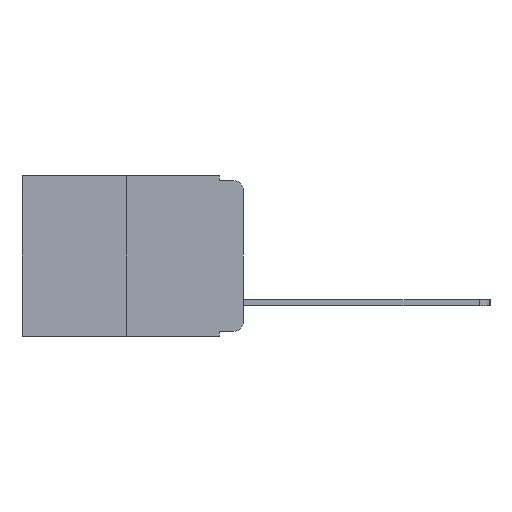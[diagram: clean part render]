
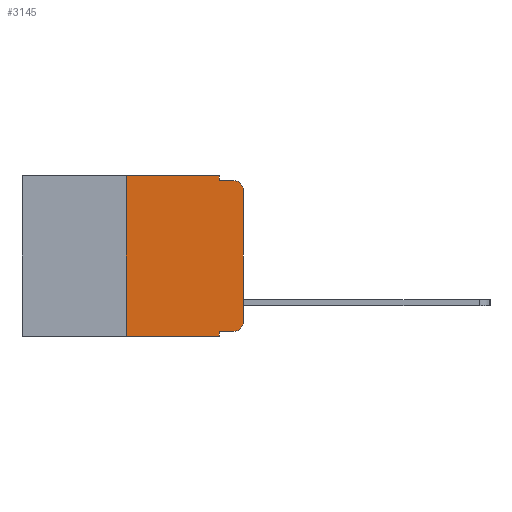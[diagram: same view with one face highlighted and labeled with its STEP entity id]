
A CAD part, left-side view. The second image highlights one B-rep face of the part: STEP entity #3145.
In plain terms, the highlighted planar face has unit normal (-1, 0, 0).
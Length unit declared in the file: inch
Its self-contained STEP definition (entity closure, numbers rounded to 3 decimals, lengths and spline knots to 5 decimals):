
#488 = VERTEX_POINT ( 'NONE', #14574 ) ;
#530 = VERTEX_POINT ( 'NONE', #11037 ) ;
#1073 = AXIS2_PLACEMENT_3D ( 'NONE', #14732, #5873, #16151 ) ;
#1412 = ORIENTED_EDGE ( 'NONE', *, *, #6481, .F. ) ;
#1425 = VECTOR ( 'NONE', #16411, 39.37008 ) ;
#1604 = DIRECTION ( 'NONE',  ( 0., -1., 0. ) ) ;
#2399 = VECTOR ( 'NONE', #10266, 39.37008 ) ;
#2474 = LINE ( 'NONE', #12346, #3529 ) ;
#2489 = VERTEX_POINT ( 'NONE', #17784 ) ;
#2563 = VECTOR ( 'NONE', #19127, 39.37008 ) ;
#2651 = AXIS2_PLACEMENT_3D ( 'NONE', #19579, #9808, #18224 ) ;
#2831 = VERTEX_POINT ( 'NONE', #5529 ) ;
#3027 = EDGE_CURVE ( 'NONE', #488, #6034, #14337, .T. ) ;
#3058 = EDGE_CURVE ( 'NONE', #14936, #2831, #10097, .T. ) ;
#3083 = DIRECTION ( 'NONE',  ( 0., 0., -1. ) ) ;
#3145 = ADVANCED_FACE ( 'NONE', ( #11165 ), #3988, .F. ) ;
#3529 = VECTOR ( 'NONE', #3083, 39.37008 ) ;
#3985 = AXIS2_PLACEMENT_3D ( 'NONE', #14388, #5452, #15778 ) ;
#3988 = PLANE ( 'NONE',  #2651 ) ;
#4686 = ORIENTED_EDGE ( 'NONE', *, *, #6106, .T. ) ;
#4803 = EDGE_CURVE ( 'NONE', #11259, #530, #14645, .T. ) ;
#5226 = LINE ( 'NONE', #15723, #12767 ) ;
#5256 = CARTESIAN_POINT ( 'NONE',  ( 0., 0.473, -0.343 ) ) ;
#5452 = DIRECTION ( 'NONE',  ( -1., 0., 0. ) ) ;
#5529 = CARTESIAN_POINT ( 'NONE',  ( 0., 0.051, -0.343 ) ) ;
#5835 = CARTESIAN_POINT ( 'NONE',  ( 0., 0.051, -0.333 ) ) ;
#5873 = DIRECTION ( 'NONE',  ( -1., 0., 0. ) ) ;
#6034 = VERTEX_POINT ( 'NONE', #12609 ) ;
#6106 = EDGE_CURVE ( 'NONE', #14936, #2489, #5226, .T. ) ;
#6107 = EDGE_CURVE ( 'NONE', #2489, #488, #16562, .T. ) ;
#6481 = EDGE_CURVE ( 'NONE', #12568, #14015, #8316, .T. ) ;
#6861 = EDGE_CURVE ( 'NONE', #6034, #14015, #16951, .T. ) ;
#6914 = DIRECTION ( 'NONE',  ( 0., -1., 0. ) ) ;
#6989 = EDGE_CURVE ( 'NONE', #11314, #11259, #10096, .T. ) ;
#7178 = CARTESIAN_POINT ( 'NONE',  ( 0., 0.473, 0. ) ) ;
#7525 = ORIENTED_EDGE ( 'NONE', *, *, #4803, .F. ) ;
#8316 = LINE ( 'NONE', #19531, #11200 ) ;
#9338 = CARTESIAN_POINT ( 'NONE',  ( 0., 0., 0. ) ) ;
#9435 = ORIENTED_EDGE ( 'NONE', *, *, #6107, .T. ) ;
#9636 = ORIENTED_EDGE ( 'NONE', *, *, #6861, .T. ) ;
#9776 = EDGE_CURVE ( 'NONE', #530, #12568, #2474, .T. ) ;
#9808 = DIRECTION ( 'NONE',  ( 1., 0., 0. ) ) ;
#10096 = LINE ( 'NONE', #15166, #17147 ) ;
#10097 = LINE ( 'NONE', #10811, #1425 ) ;
#10266 = DIRECTION ( 'NONE',  ( 0., -1., 0. ) ) ;
#10811 = CARTESIAN_POINT ( 'NONE',  ( 0., 0.051, 0. ) ) ;
#11037 = CARTESIAN_POINT ( 'NONE',  ( 0., 0.051, 0. ) ) ;
#11165 = FACE_OUTER_BOUND ( 'NONE', #12363, .T. ) ;
#11173 = VECTOR ( 'NONE', #6914, 39.37008 ) ;
#11200 = VECTOR ( 'NONE', #1604, 39.37008 ) ;
#11259 = VERTEX_POINT ( 'NONE', #12084 ) ;
#11314 = VERTEX_POINT ( 'NONE', #15027 ) ;
#12084 = CARTESIAN_POINT ( 'NONE',  ( 0., 0.25, 0. ) ) ;
#12289 = ORIENTED_EDGE ( 'NONE', *, *, #3058, .F. ) ;
#12346 = CARTESIAN_POINT ( 'NONE',  ( 0., 0.051, 0. ) ) ;
#12363 = EDGE_LOOP ( 'NONE', ( #16311, #9636, #1412, #17996, #7525, #15209, #19276, #12289, #4686, #9435 ) ) ;
#12568 = VERTEX_POINT ( 'NONE', #15909 ) ;
#12609 = CARTESIAN_POINT ( 'NONE',  ( 0., 0., -0.03 ) ) ;
#12767 = VECTOR ( 'NONE', #14328, 39.37008 ) ;
#14015 = VERTEX_POINT ( 'NONE', #14419 ) ;
#14328 = DIRECTION ( 'NONE',  ( 0., -1., 0. ) ) ;
#14337 = LINE ( 'NONE', #9338, #2563 ) ;
#14388 = CARTESIAN_POINT ( 'NONE',  ( 0., 0.02, -0.313 ) ) ;
#14419 = CARTESIAN_POINT ( 'NONE',  ( 0., 0.02, -0.01 ) ) ;
#14574 = CARTESIAN_POINT ( 'NONE',  ( 0., 0., -0.313 ) ) ;
#14617 = EDGE_CURVE ( 'NONE', #11314, #2831, #14999, .T. ) ;
#14645 = LINE ( 'NONE', #7178, #2399 ) ;
#14732 = CARTESIAN_POINT ( 'NONE',  ( 0., 0.02, -0.03 ) ) ;
#14936 = VERTEX_POINT ( 'NONE', #5835 ) ;
#14999 = LINE ( 'NONE', #5256, #11173 ) ;
#15027 = CARTESIAN_POINT ( 'NONE',  ( 0., 0.25, -0.343 ) ) ;
#15166 = CARTESIAN_POINT ( 'NONE',  ( 0., 0.25, 0. ) ) ;
#15209 = ORIENTED_EDGE ( 'NONE', *, *, #6989, .F. ) ;
#15723 = CARTESIAN_POINT ( 'NONE',  ( 0., 0.051, -0.333 ) ) ;
#15778 = DIRECTION ( 'NONE',  ( 0., 0., -1. ) ) ;
#15909 = CARTESIAN_POINT ( 'NONE',  ( 0., 0.051, -0.01 ) ) ;
#16151 = DIRECTION ( 'NONE',  ( 0., 0., -1. ) ) ;
#16311 = ORIENTED_EDGE ( 'NONE', *, *, #3027, .T. ) ;
#16411 = DIRECTION ( 'NONE',  ( 0., 0., -1. ) ) ;
#16562 = CIRCLE ( 'NONE', #3985, 0.02 ) ;
#16577 = DIRECTION ( 'NONE',  ( 0., 0., 1. ) ) ;
#16951 = CIRCLE ( 'NONE', #1073, 0.02 ) ;
#17147 = VECTOR ( 'NONE', #16577, 39.37008 ) ;
#17784 = CARTESIAN_POINT ( 'NONE',  ( 0., 0.02, -0.333 ) ) ;
#17996 = ORIENTED_EDGE ( 'NONE', *, *, #9776, .F. ) ;
#18224 = DIRECTION ( 'NONE',  ( 0., 0., -1. ) ) ;
#19127 = DIRECTION ( 'NONE',  ( 0., 0., 1. ) ) ;
#19276 = ORIENTED_EDGE ( 'NONE', *, *, #14617, .T. ) ;
#19531 = CARTESIAN_POINT ( 'NONE',  ( 0., 0.051, -0.01 ) ) ;
#19579 = CARTESIAN_POINT ( 'NONE',  ( 0., 0.473, 0. ) ) ;
